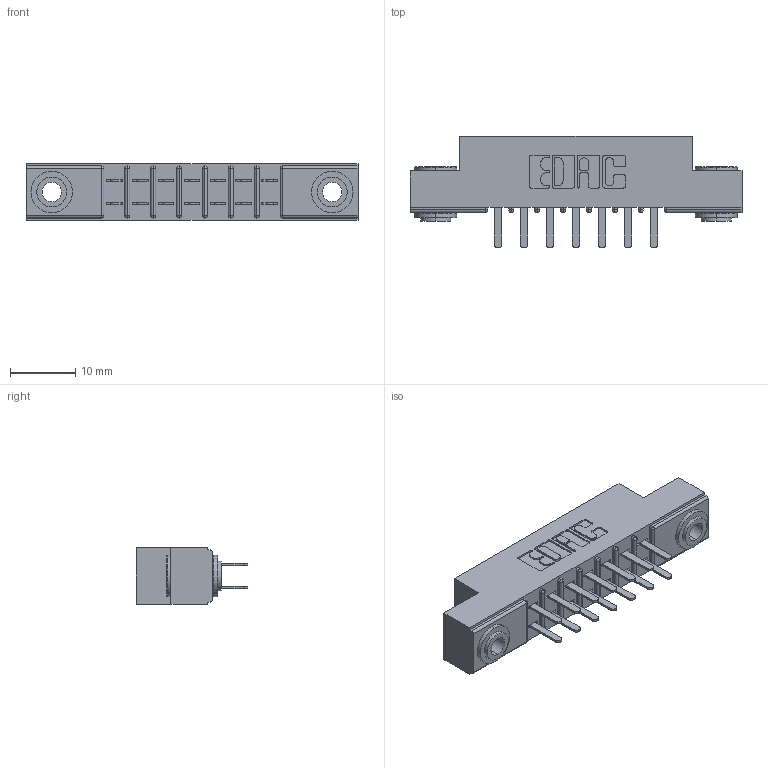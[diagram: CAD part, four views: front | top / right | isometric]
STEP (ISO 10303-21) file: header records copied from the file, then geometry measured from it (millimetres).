
FILE_DESCRIPTION (( 'STEP AP203' ), '1' );
FILE_NAME ('305-014-520-503.STEP', '2019-09-09T11:45:49', ( '' ), ( '' ), 'SwSTEP 2.0', 'SolidWorks 2016', '' );
FILE_SCHEMA (( 'CONFIG_CONTROL_DESIGN' ));
Length unit declared in the file: inch
Products named in the file (4): 305-014-520-503; 305 Part_.156 Dia; 345-250-002_345-250-002-102; 305-290-001_520
Assembly tree (17 placements, depth 2):
  305-014-520-503
    305 Part_.156 Dia
    305-290-001_520  x14
    345-250-002_345-250-002-102  x2
Bounding box: 50.75 x 17.09 x 8.71 mm (x, y, z)
Volume: 3100.5 mm3; surface area: 5473 mm2
Topology: 17 solids, 17 shells, 812 faces, 2269 edges, 1470 vertices
Faces by surface type: plane 470, cylinder 306, sphere 28, cone 8
Entity records: 12785 total; most frequent: CARTESIAN_POINT 2096, DIRECTION 2071, ORIENTED_EDGE 2066, EDGE_CURVE 1033, LINE 789, VECTOR 789, VERTEX_POINT 666, AXIS2_PLACEMENT_3D 641
